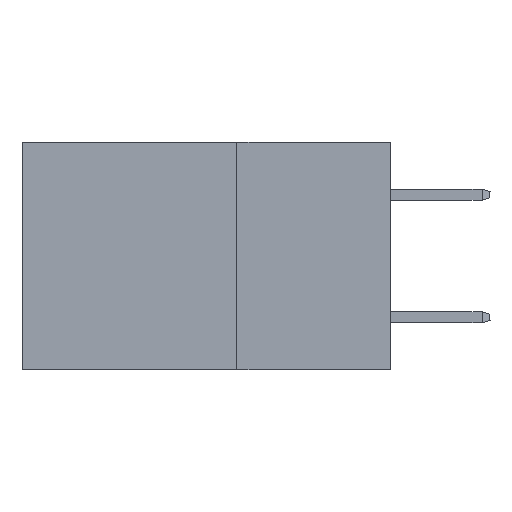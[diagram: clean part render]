
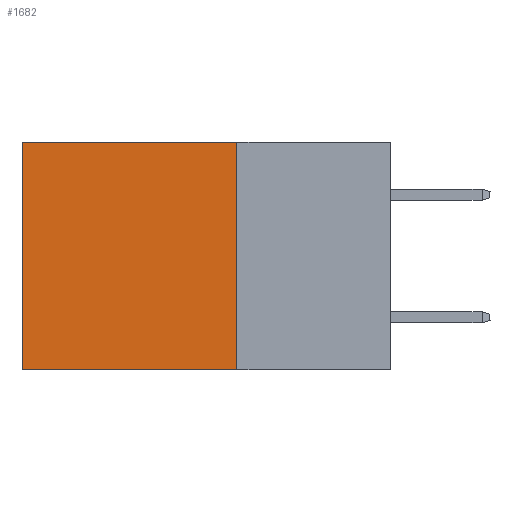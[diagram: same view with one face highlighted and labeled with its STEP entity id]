
A CAD part, left-side view. The second image highlights one B-rep face of the part: STEP entity #1682.
In plain terms, the highlighted planar face has unit normal (-1, 0, 0).
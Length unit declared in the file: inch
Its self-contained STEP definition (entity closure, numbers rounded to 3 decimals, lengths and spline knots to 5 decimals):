
#625 = CARTESIAN_POINT ( 'NONE',  ( 0.2875, 0.25, -0.37 ) ) ;
#785 = CARTESIAN_POINT ( 'NONE',  ( 0.2875, 0.25, 0. ) ) ;
#962 = CARTESIAN_POINT ( 'NONE',  ( 0.2875, 0.6, -0.37 ) ) ;
#1682 = ADVANCED_FACE ( 'NONE', ( #33149 ), #8595, .F. ) ;
#2409 = EDGE_LOOP ( 'NONE', ( #27451, #5819, #10822, #33664 ) ) ;
#3943 = CARTESIAN_POINT ( 'NONE',  ( 0.2875, 0.25, 0. ) ) ;
#4656 = LINE ( 'NONE', #3943, #33949 ) ;
#5819 = ORIENTED_EDGE ( 'NONE', *, *, #31624, .F. ) ;
#6688 = DIRECTION ( 'NONE',  ( 0., 0., -1. ) ) ;
#8595 = PLANE ( 'NONE',  #26245 ) ;
#10822 = ORIENTED_EDGE ( 'NONE', *, *, #23718, .F. ) ;
#12987 = DIRECTION ( 'NONE',  ( 0., 1., 0. ) ) ;
#14381 = DIRECTION ( 'NONE',  ( 0., 0., -1. ) ) ;
#16283 = LINE ( 'NONE', #18576, #30472 ) ;
#16425 = EDGE_CURVE ( 'NONE', #17085, #20410, #35679, .T. ) ;
#17085 = VERTEX_POINT ( 'NONE', #23173 ) ;
#17279 = DIRECTION ( 'NONE',  ( 0., 0., -1. ) ) ;
#17996 = VECTOR ( 'NONE', #17279, 39.37008 ) ;
#18576 = CARTESIAN_POINT ( 'NONE',  ( 0.2875, 0.25, -0.37 ) ) ;
#18758 = CARTESIAN_POINT ( 'NONE',  ( 0.2875, 0.25, 0. ) ) ;
#19702 = VERTEX_POINT ( 'NONE', #625 ) ;
#20410 = VERTEX_POINT ( 'NONE', #962 ) ;
#22848 = CARTESIAN_POINT ( 'NONE',  ( 0.2875, 0.6, 0. ) ) ;
#23173 = CARTESIAN_POINT ( 'NONE',  ( 0.2875, 0.6, 0. ) ) ;
#23718 = EDGE_CURVE ( 'NONE', #25555, #19702, #4656, .T. ) ;
#25555 = VERTEX_POINT ( 'NONE', #785 ) ;
#26245 = AXIS2_PLACEMENT_3D ( 'NONE', #28534, #31364, #14381 ) ;
#27290 = EDGE_CURVE ( 'NONE', #25555, #17085, #29426, .T. ) ;
#27451 = ORIENTED_EDGE ( 'NONE', *, *, #16425, .T. ) ;
#28534 = CARTESIAN_POINT ( 'NONE',  ( 0.2875, 0.25, 0. ) ) ;
#29426 = LINE ( 'NONE', #18758, #36027 ) ;
#30472 = VECTOR ( 'NONE', #32666, 39.37008 ) ;
#31364 = DIRECTION ( 'NONE',  ( 1., 0., 0. ) ) ;
#31624 = EDGE_CURVE ( 'NONE', #19702, #20410, #16283, .T. ) ;
#32666 = DIRECTION ( 'NONE',  ( 0., 1., 0. ) ) ;
#33149 = FACE_OUTER_BOUND ( 'NONE', #2409, .T. ) ;
#33664 = ORIENTED_EDGE ( 'NONE', *, *, #27290, .T. ) ;
#33949 = VECTOR ( 'NONE', #6688, 39.37008 ) ;
#35679 = LINE ( 'NONE', #22848, #17996 ) ;
#36027 = VECTOR ( 'NONE', #12987, 39.37008 ) ;
